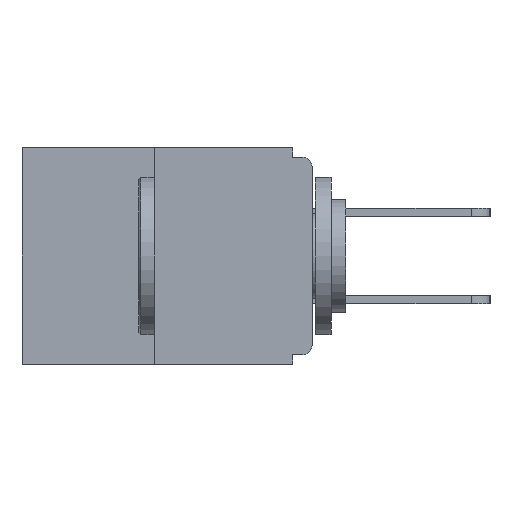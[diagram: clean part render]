
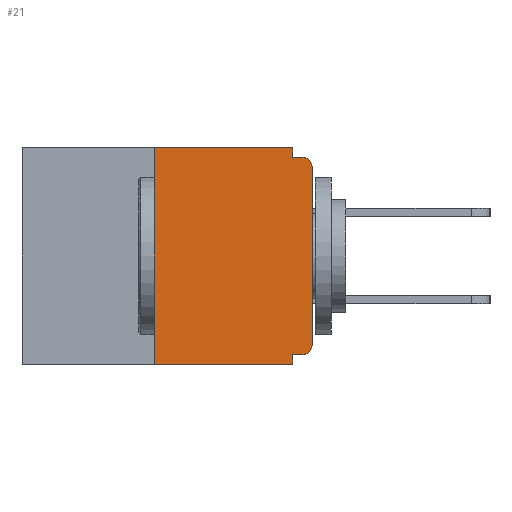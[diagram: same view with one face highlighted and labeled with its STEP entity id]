
A CAD part, left-side view. The second image highlights one B-rep face of the part: STEP entity #21.
In plain terms, the highlighted planar face has unit normal (-1, 0, 0).
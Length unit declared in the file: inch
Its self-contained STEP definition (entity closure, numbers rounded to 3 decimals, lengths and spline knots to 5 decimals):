
#21 = ADVANCED_FACE ( 'NONE', ( #21378 ), #24019, .F. ) ;
#754 = EDGE_LOOP ( 'NONE', ( #22681, #1898, #15904, #2770, #16361, #6509, #4726, #16936, #22057, #20045 ) ) ;
#927 = VECTOR ( 'NONE', #9049, 39.37008 ) ;
#1062 = CARTESIAN_POINT ( 'NONE',  ( 0., 0.031, -0.328 ) ) ;
#1252 = DIRECTION ( 'NONE',  ( 0., -1., 0. ) ) ;
#1879 = DIRECTION ( 'NONE',  ( 0., 0., 1. ) ) ;
#1898 = ORIENTED_EDGE ( 'NONE', *, *, #1922, .F. ) ;
#1912 = DIRECTION ( 'NONE',  ( 0., 0., -1. ) ) ;
#1922 = EDGE_CURVE ( 'NONE', #10613, #8890, #6500, .T. ) ;
#2244 = DIRECTION ( 'NONE',  ( -1., 0., 0. ) ) ;
#2764 = VERTEX_POINT ( 'NONE', #9533 ) ;
#2770 = ORIENTED_EDGE ( 'NONE', *, *, #22272, .F. ) ;
#3565 = LINE ( 'NONE', #8562, #8013 ) ;
#4325 = DIRECTION ( 'NONE',  ( -1., 0., 0. ) ) ;
#4365 = CARTESIAN_POINT ( 'NONE',  ( 0., 0.031, -0.343 ) ) ;
#4462 = VECTOR ( 'NONE', #9648, 39.37008 ) ;
#4726 = ORIENTED_EDGE ( 'NONE', *, *, #13399, .T. ) ;
#5208 = CARTESIAN_POINT ( 'NONE',  ( 0., 0., -0.015 ) ) ;
#5697 = VERTEX_POINT ( 'NONE', #8980 ) ;
#6466 = VECTOR ( 'NONE', #12052, 39.37008 ) ;
#6500 = LINE ( 'NONE', #14624, #20405 ) ;
#6509 = ORIENTED_EDGE ( 'NONE', *, *, #9873, .T. ) ;
#6538 = AXIS2_PLACEMENT_3D ( 'NONE', #13923, #4325, #8220 ) ;
#6954 = EDGE_CURVE ( 'NONE', #2764, #14610, #10390, .T. ) ;
#7884 = CIRCLE ( 'NONE', #6538, 0.015 ) ;
#8013 = VECTOR ( 'NONE', #17810, 39.37008 ) ;
#8220 = DIRECTION ( 'NONE',  ( 0., 0., -1. ) ) ;
#8562 = CARTESIAN_POINT ( 'NONE',  ( 0., 0.031, -0.343 ) ) ;
#8890 = VERTEX_POINT ( 'NONE', #9444 ) ;
#8980 = CARTESIAN_POINT ( 'NONE',  ( 0., 0.015, -0.015 ) ) ;
#9049 = DIRECTION ( 'NONE',  ( 0., 1., 0. ) ) ;
#9306 = AXIS2_PLACEMENT_3D ( 'NONE', #13418, #2244, #1912 ) ;
#9444 = CARTESIAN_POINT ( 'NONE',  ( 0., 0.25, 0. ) ) ;
#9533 = CARTESIAN_POINT ( 'NONE',  ( 0., 0.031, 0. ) ) ;
#9537 = CARTESIAN_POINT ( 'NONE',  ( 0., 0.031, 0. ) ) ;
#9648 = DIRECTION ( 'NONE',  ( 0., -1., 0. ) ) ;
#9873 = EDGE_CURVE ( 'NONE', #13283, #20374, #7884, .T. ) ;
#10390 = LINE ( 'NONE', #9537, #12464 ) ;
#10401 = CARTESIAN_POINT ( 'NONE',  ( 0., 0., -0.03 ) ) ;
#10613 = VERTEX_POINT ( 'NONE', #23607 ) ;
#10712 = CIRCLE ( 'NONE', #9306, 0.015 ) ;
#10739 = AXIS2_PLACEMENT_3D ( 'NONE', #14445, #12703, #16261 ) ;
#11563 = LINE ( 'NONE', #15197, #4462 ) ;
#11956 = EDGE_CURVE ( 'NONE', #14610, #5697, #14221, .T. ) ;
#12052 = DIRECTION ( 'NONE',  ( 0., 0., 1. ) ) ;
#12464 = VECTOR ( 'NONE', #15253, 39.37008 ) ;
#12703 = DIRECTION ( 'NONE',  ( 1., 0., 0. ) ) ;
#12765 = LINE ( 'NONE', #18530, #927 ) ;
#13283 = VERTEX_POINT ( 'NONE', #15940 ) ;
#13399 = EDGE_CURVE ( 'NONE', #20374, #14760, #13577, .T. ) ;
#13418 = CARTESIAN_POINT ( 'NONE',  ( 0., 0.015, -0.03 ) ) ;
#13577 = LINE ( 'NONE', #21552, #6466 ) ;
#13923 = CARTESIAN_POINT ( 'NONE',  ( 0., 0.015, -0.313 ) ) ;
#14125 = VECTOR ( 'NONE', #22761, 39.37008 ) ;
#14221 = LINE ( 'NONE', #5208, #16857 ) ;
#14445 = CARTESIAN_POINT ( 'NONE',  ( 0., 0.46, 0. ) ) ;
#14610 = VERTEX_POINT ( 'NONE', #23305 ) ;
#14624 = CARTESIAN_POINT ( 'NONE',  ( 0., 0.25, 0. ) ) ;
#14760 = VERTEX_POINT ( 'NONE', #10401 ) ;
#15197 = CARTESIAN_POINT ( 'NONE',  ( 0., 0.46, -0.343 ) ) ;
#15253 = DIRECTION ( 'NONE',  ( 0., 0., -1. ) ) ;
#15904 = ORIENTED_EDGE ( 'NONE', *, *, #22073, .T. ) ;
#15940 = CARTESIAN_POINT ( 'NONE',  ( 0., 0.015, -0.328 ) ) ;
#16261 = DIRECTION ( 'NONE',  ( 0., 0., -1. ) ) ;
#16361 = ORIENTED_EDGE ( 'NONE', *, *, #21624, .F. ) ;
#16371 = VERTEX_POINT ( 'NONE', #4365 ) ;
#16857 = VECTOR ( 'NONE', #1252, 39.37008 ) ;
#16936 = ORIENTED_EDGE ( 'NONE', *, *, #17360, .T. ) ;
#17360 = EDGE_CURVE ( 'NONE', #14760, #5697, #10712, .T. ) ;
#17810 = DIRECTION ( 'NONE',  ( 0., 0., -1. ) ) ;
#18530 = CARTESIAN_POINT ( 'NONE',  ( 0., 0., -0.328 ) ) ;
#18551 = EDGE_CURVE ( 'NONE', #8890, #2764, #20649, .T. ) ;
#18966 = VERTEX_POINT ( 'NONE', #1062 ) ;
#20045 = ORIENTED_EDGE ( 'NONE', *, *, #6954, .F. ) ;
#20174 = CARTESIAN_POINT ( 'NONE',  ( 0., 0., -0.313 ) ) ;
#20374 = VERTEX_POINT ( 'NONE', #20174 ) ;
#20405 = VECTOR ( 'NONE', #1879, 39.37008 ) ;
#20649 = LINE ( 'NONE', #20883, #14125 ) ;
#20883 = CARTESIAN_POINT ( 'NONE',  ( 0., 0.46, 0. ) ) ;
#21378 = FACE_OUTER_BOUND ( 'NONE', #754, .T. ) ;
#21552 = CARTESIAN_POINT ( 'NONE',  ( 0., 0., 0. ) ) ;
#21624 = EDGE_CURVE ( 'NONE', #13283, #18966, #12765, .T. ) ;
#22057 = ORIENTED_EDGE ( 'NONE', *, *, #11956, .F. ) ;
#22073 = EDGE_CURVE ( 'NONE', #10613, #16371, #11563, .T. ) ;
#22272 = EDGE_CURVE ( 'NONE', #18966, #16371, #3565, .T. ) ;
#22681 = ORIENTED_EDGE ( 'NONE', *, *, #18551, .F. ) ;
#22761 = DIRECTION ( 'NONE',  ( 0., -1., 0. ) ) ;
#23305 = CARTESIAN_POINT ( 'NONE',  ( 0., 0.031, -0.015 ) ) ;
#23607 = CARTESIAN_POINT ( 'NONE',  ( 0., 0.25, -0.343 ) ) ;
#24019 = PLANE ( 'NONE',  #10739 ) ;
